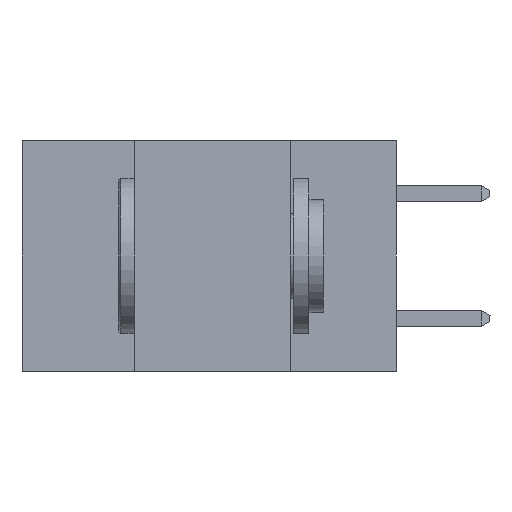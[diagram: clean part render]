
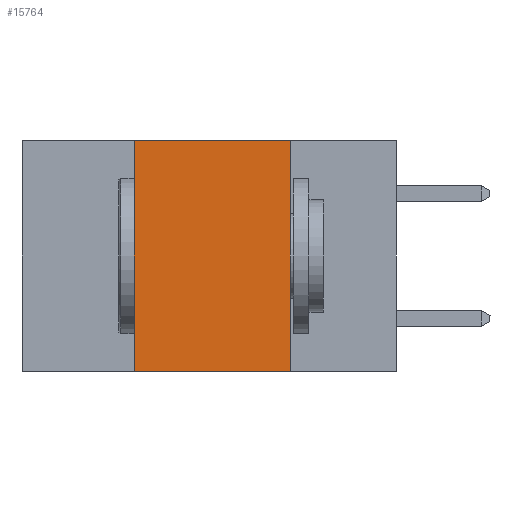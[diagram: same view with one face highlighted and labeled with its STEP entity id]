
A CAD part, left-side view. The second image highlights one B-rep face of the part: STEP entity #15764.
In plain terms, the highlighted planar face has unit normal (-1, 0, 0).
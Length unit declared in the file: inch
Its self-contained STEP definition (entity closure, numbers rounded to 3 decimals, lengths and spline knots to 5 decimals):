
#2612 = PLANE ( 'NONE',  #17955 ) ;
#2750 = DIRECTION ( 'NONE',  ( 1., 0., 0. ) ) ;
#3801 = LINE ( 'NONE', #17782, #19602 ) ;
#4101 = CARTESIAN_POINT ( 'NONE',  ( 0., 0.17, 0. ) ) ;
#4556 = DIRECTION ( 'NONE',  ( 0., 0., 1. ) ) ;
#5333 = VERTEX_POINT ( 'NONE', #9856 ) ;
#5615 = ORIENTED_EDGE ( 'NONE', *, *, #17491, .F. ) ;
#5707 = EDGE_CURVE ( 'NONE', #12821, #9501, #7875, .T. ) ;
#6672 = DIRECTION ( 'NONE',  ( 0., 0., -1. ) ) ;
#7331 = DIRECTION ( 'NONE',  ( 0., 0., -1. ) ) ;
#7660 = EDGE_CURVE ( 'NONE', #5333, #15272, #3801, .T. ) ;
#7729 = CARTESIAN_POINT ( 'NONE',  ( 0., 0.6, 0. ) ) ;
#7875 = LINE ( 'NONE', #7729, #16974 ) ;
#8102 = EDGE_CURVE ( 'NONE', #9501, #15272, #11863, .T. ) ;
#9219 = LINE ( 'NONE', #12193, #19792 ) ;
#9229 = FACE_OUTER_BOUND ( 'NONE', #10413, .T. ) ;
#9501 = VERTEX_POINT ( 'NONE', #4101 ) ;
#9856 = CARTESIAN_POINT ( 'NONE',  ( 0., 0.42, -0.37 ) ) ;
#10413 = EDGE_LOOP ( 'NONE', ( #18376, #13173, #5615, #18639 ) ) ;
#11633 = CARTESIAN_POINT ( 'NONE',  ( 0., 0.17, -0.37 ) ) ;
#11863 = LINE ( 'NONE', #15709, #13590 ) ;
#12193 = CARTESIAN_POINT ( 'NONE',  ( 0., 0.42, 0. ) ) ;
#12821 = VERTEX_POINT ( 'NONE', #15104 ) ;
#13173 = ORIENTED_EDGE ( 'NONE', *, *, #5707, .F. ) ;
#13288 = CARTESIAN_POINT ( 'NONE',  ( 0., 0.6, 0. ) ) ;
#13590 = VECTOR ( 'NONE', #6672, 39.37008 ) ;
#15104 = CARTESIAN_POINT ( 'NONE',  ( 0., 0.42, 0. ) ) ;
#15272 = VERTEX_POINT ( 'NONE', #11633 ) ;
#15709 = CARTESIAN_POINT ( 'NONE',  ( 0., 0.17, 0. ) ) ;
#15764 = ADVANCED_FACE ( 'NONE', ( #9229 ), #2612, .F. ) ;
#16974 = VECTOR ( 'NONE', #18323, 39.37008 ) ;
#17491 = EDGE_CURVE ( 'NONE', #5333, #12821, #9219, .T. ) ;
#17782 = CARTESIAN_POINT ( 'NONE',  ( 0., 0.6, -0.37 ) ) ;
#17913 = DIRECTION ( 'NONE',  ( 0., -1., 0. ) ) ;
#17955 = AXIS2_PLACEMENT_3D ( 'NONE', #13288, #2750, #7331 ) ;
#18323 = DIRECTION ( 'NONE',  ( 0., -1., 0. ) ) ;
#18376 = ORIENTED_EDGE ( 'NONE', *, *, #8102, .F. ) ;
#18639 = ORIENTED_EDGE ( 'NONE', *, *, #7660, .T. ) ;
#19602 = VECTOR ( 'NONE', #17913, 39.37008 ) ;
#19792 = VECTOR ( 'NONE', #4556, 39.37008 ) ;
